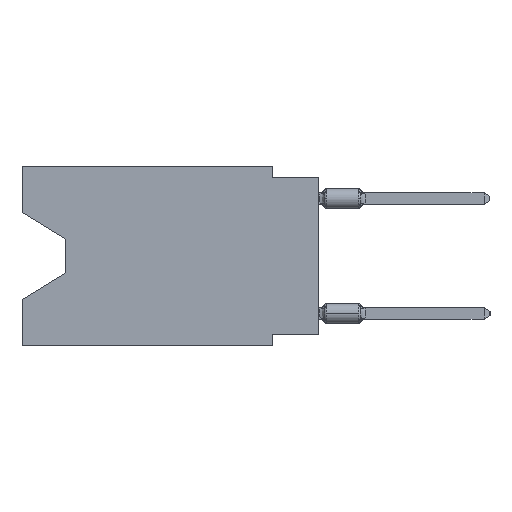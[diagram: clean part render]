
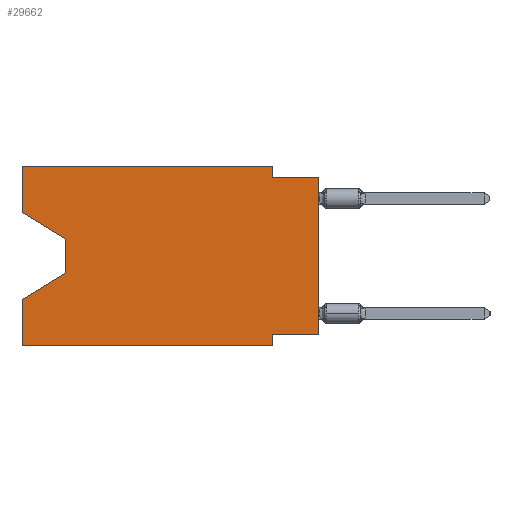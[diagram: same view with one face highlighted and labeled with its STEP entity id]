
A CAD part, left-side view. The second image highlights one B-rep face of the part: STEP entity #29662.
In plain terms, the highlighted planar face has unit normal (-1, 0, 0).
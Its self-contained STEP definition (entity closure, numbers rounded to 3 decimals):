
#4 = CARTESIAN_POINT ( 'NONE',  ( 0., 16.383, -2.546 ) ) ;
#135 = EDGE_CURVE ( 'NONE', #339, #26755, #7761, .T. ) ;
#339 = VERTEX_POINT ( 'NONE', #7620 ) ;
#479 = ORIENTED_EDGE ( 'NONE', *, *, #25943, .F. ) ;
#1048 = DIRECTION ( 'NONE',  ( 0., 0., 1. ) ) ;
#1621 = CARTESIAN_POINT ( 'NONE',  ( 0., 2.54, 0. ) ) ;
#1656 = CARTESIAN_POINT ( 'NONE',  ( 0., 0., -0.635 ) ) ;
#1829 = VERTEX_POINT ( 'NONE', #8906 ) ;
#2069 = EDGE_CURVE ( 'NONE', #29042, #1829, #21706, .T. ) ;
#2157 = EDGE_CURVE ( 'NONE', #2559, #8775, #18395, .T. ) ;
#2547 = ORIENTED_EDGE ( 'NONE', *, *, #8610, .F. ) ;
#2559 = VERTEX_POINT ( 'NONE', #4 ) ;
#2670 = VERTEX_POINT ( 'NONE', #23765 ) ;
#2884 = LINE ( 'NONE', #12182, #27381 ) ;
#4841 = DIRECTION ( 'NONE',  ( 0., 0., 1. ) ) ;
#5293 = AXIS2_PLACEMENT_3D ( 'NONE', #22573, #20767, #25440 ) ;
#6668 = CARTESIAN_POINT ( 'NONE',  ( 0., 13.97, -5.893 ) ) ;
#6730 = EDGE_CURVE ( 'NONE', #26755, #2670, #29600, .T. ) ;
#6998 = DIRECTION ( 'NONE',  ( 0., 0., -1. ) ) ;
#7207 = CARTESIAN_POINT ( 'NONE',  ( 0., 2.54, -9.906 ) ) ;
#7317 = CARTESIAN_POINT ( 'NONE',  ( 0., 16.383, -2.546 ) ) ;
#7439 = CARTESIAN_POINT ( 'NONE',  ( 0., 0., -9.271 ) ) ;
#7620 = CARTESIAN_POINT ( 'NONE',  ( 0., 13.97, -4.013 ) ) ;
#7761 = LINE ( 'NONE', #23293, #10904 ) ;
#8610 = EDGE_CURVE ( 'NONE', #29449, #2670, #2884, .T. ) ;
#8775 = VERTEX_POINT ( 'NONE', #11242 ) ;
#8906 = CARTESIAN_POINT ( 'NONE',  ( 0., 0., -0.635 ) ) ;
#8987 = CARTESIAN_POINT ( 'NONE',  ( 0., 2.54, -9.271 ) ) ;
#9450 = CARTESIAN_POINT ( 'NONE',  ( 0., 16.383, -9.906 ) ) ;
#9551 = ORIENTED_EDGE ( 'NONE', *, *, #11568, .F. ) ;
#9946 = DIRECTION ( 'NONE',  ( 0., 0., 1. ) ) ;
#10202 = VECTOR ( 'NONE', #24618, 1000. ) ;
#10570 = LINE ( 'NONE', #7317, #10760 ) ;
#10680 = CARTESIAN_POINT ( 'NONE',  ( 0., 0., 0. ) ) ;
#10760 = VECTOR ( 'NONE', #17029, 1000. ) ;
#10904 = VECTOR ( 'NONE', #16932, 1000. ) ;
#10943 = VECTOR ( 'NONE', #11479, 1000. ) ;
#11008 = EDGE_CURVE ( 'NONE', #29042, #13507, #23104, .T. ) ;
#11208 = PLANE ( 'NONE',  #5293 ) ;
#11242 = CARTESIAN_POINT ( 'NONE',  ( 0., 16.383, 0. ) ) ;
#11479 = DIRECTION ( 'NONE',  ( 0., 0.855, -0.519 ) ) ;
#11568 = EDGE_CURVE ( 'NONE', #13986, #1829, #25629, .T. ) ;
#11635 = DIRECTION ( 'NONE',  ( 0., 1., 0. ) ) ;
#12182 = CARTESIAN_POINT ( 'NONE',  ( 0., 16.383, 0. ) ) ;
#12339 = CARTESIAN_POINT ( 'NONE',  ( 0., 2.54, 0. ) ) ;
#12342 = CARTESIAN_POINT ( 'NONE',  ( 0., 16.383, 0. ) ) ;
#12872 = ORIENTED_EDGE ( 'NONE', *, *, #2157, .F. ) ;
#13507 = VERTEX_POINT ( 'NONE', #8987 ) ;
#13657 = ORIENTED_EDGE ( 'NONE', *, *, #135, .T. ) ;
#13986 = VERTEX_POINT ( 'NONE', #19021 ) ;
#14109 = VECTOR ( 'NONE', #26942, 1000. ) ;
#14960 = VERTEX_POINT ( 'NONE', #12339 ) ;
#15078 = DIRECTION ( 'NONE',  ( 0., -1., 0. ) ) ;
#15484 = EDGE_CURVE ( 'NONE', #13507, #25608, #20575, .T. ) ;
#15845 = CARTESIAN_POINT ( 'NONE',  ( 0., 16.383, 0. ) ) ;
#16183 = VECTOR ( 'NONE', #22289, 1000. ) ;
#16186 = EDGE_CURVE ( 'NONE', #8775, #14960, #17178, .T. ) ;
#16687 = CARTESIAN_POINT ( 'NONE',  ( 0., 16.383, -9.906 ) ) ;
#16932 = DIRECTION ( 'NONE',  ( 0., 0., -1. ) ) ;
#16948 = EDGE_CURVE ( 'NONE', #29449, #25608, #18799, .T. ) ;
#17029 = DIRECTION ( 'NONE',  ( 0., -0.855, -0.519 ) ) ;
#17178 = LINE ( 'NONE', #12342, #24610 ) ;
#17719 = LINE ( 'NONE', #1621, #14109 ) ;
#17724 = ORIENTED_EDGE ( 'NONE', *, *, #6730, .T. ) ;
#17916 = CARTESIAN_POINT ( 'NONE',  ( 0., 13.97, -5.893 ) ) ;
#18395 = LINE ( 'NONE', #15845, #24746 ) ;
#18413 = ORIENTED_EDGE ( 'NONE', *, *, #11008, .F. ) ;
#18799 = LINE ( 'NONE', #9450, #10202 ) ;
#19021 = CARTESIAN_POINT ( 'NONE',  ( 0., 2.54, -0.635 ) ) ;
#19255 = EDGE_LOOP ( 'NONE', ( #28641, #13657, #17724, #2547, #19939, #20460, #18413, #26943, #9551, #479, #21907, #12872 ) ) ;
#19939 = ORIENTED_EDGE ( 'NONE', *, *, #16948, .T. ) ;
#20460 = ORIENTED_EDGE ( 'NONE', *, *, #15484, .F. ) ;
#20575 = LINE ( 'NONE', #25245, #25074 ) ;
#20767 = DIRECTION ( 'NONE',  ( 1., 0., 0. ) ) ;
#21706 = LINE ( 'NONE', #10680, #21866 ) ;
#21866 = VECTOR ( 'NONE', #1048, 1000. ) ;
#21907 = ORIENTED_EDGE ( 'NONE', *, *, #16186, .F. ) ;
#22289 = DIRECTION ( 'NONE',  ( 0., -1., 0. ) ) ;
#22573 = CARTESIAN_POINT ( 'NONE',  ( 0., 16.383, 0. ) ) ;
#23104 = LINE ( 'NONE', #24914, #26477 ) ;
#23293 = CARTESIAN_POINT ( 'NONE',  ( 0., 13.97, -4.013 ) ) ;
#23765 = CARTESIAN_POINT ( 'NONE',  ( 0., 16.383, -7.36 ) ) ;
#24610 = VECTOR ( 'NONE', #15078, 1000. ) ;
#24618 = DIRECTION ( 'NONE',  ( 0., -1., 0. ) ) ;
#24746 = VECTOR ( 'NONE', #4841, 1000. ) ;
#24914 = CARTESIAN_POINT ( 'NONE',  ( 0., 0., -9.271 ) ) ;
#25074 = VECTOR ( 'NONE', #6998, 1000. ) ;
#25245 = CARTESIAN_POINT ( 'NONE',  ( 0., 2.54, -9.906 ) ) ;
#25440 = DIRECTION ( 'NONE',  ( 0., 0., -1. ) ) ;
#25608 = VERTEX_POINT ( 'NONE', #7207 ) ;
#25629 = LINE ( 'NONE', #1656, #16183 ) ;
#25943 = EDGE_CURVE ( 'NONE', #14960, #13986, #17719, .T. ) ;
#26159 = EDGE_CURVE ( 'NONE', #2559, #339, #10570, .T. ) ;
#26477 = VECTOR ( 'NONE', #11635, 1000. ) ;
#26755 = VERTEX_POINT ( 'NONE', #17916 ) ;
#26942 = DIRECTION ( 'NONE',  ( 0., 0., -1. ) ) ;
#26943 = ORIENTED_EDGE ( 'NONE', *, *, #2069, .T. ) ;
#27381 = VECTOR ( 'NONE', #9946, 1000. ) ;
#27861 = FACE_OUTER_BOUND ( 'NONE', #19255, .T. ) ;
#28641 = ORIENTED_EDGE ( 'NONE', *, *, #26159, .T. ) ;
#29042 = VERTEX_POINT ( 'NONE', #7439 ) ;
#29449 = VERTEX_POINT ( 'NONE', #16687 ) ;
#29600 = LINE ( 'NONE', #6668, #10943 ) ;
#29662 = ADVANCED_FACE ( 'NONE', ( #27861 ), #11208, .F. ) ;
